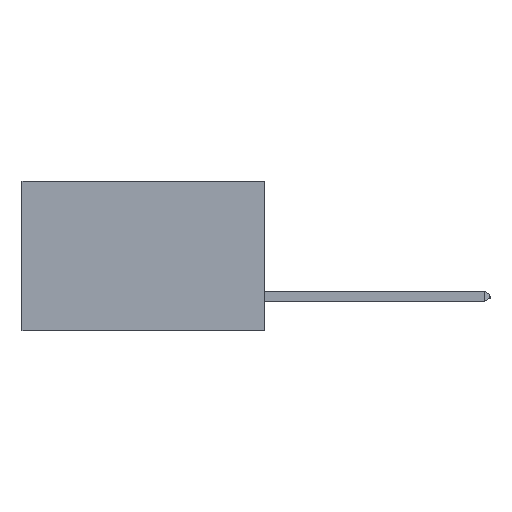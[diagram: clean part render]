
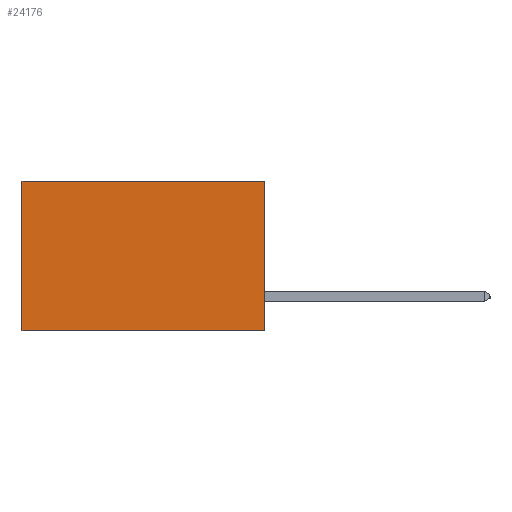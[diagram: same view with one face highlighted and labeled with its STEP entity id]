
A CAD part, left-side view. The second image highlights one B-rep face of the part: STEP entity #24176.
In plain terms, the highlighted planar face has unit normal (-1, 0, 0).
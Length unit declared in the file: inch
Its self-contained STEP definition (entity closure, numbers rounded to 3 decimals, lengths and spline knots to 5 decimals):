
#1986 = DIRECTION ( 'NONE',  ( 0., 0., -1. ) ) ;
#2754 = FACE_OUTER_BOUND ( 'NONE', #14046, .T. ) ;
#4395 = EDGE_CURVE ( 'NONE', #18801, #5040, #16166, .T. ) ;
#4834 = VERTEX_POINT ( 'NONE', #11381 ) ;
#5012 = AXIS2_PLACEMENT_3D ( 'NONE', #21224, #13677, #1986 ) ;
#5040 = VERTEX_POINT ( 'NONE', #22169 ) ;
#5149 = CARTESIAN_POINT ( 'NONE',  ( 0.298, 0., 0. ) ) ;
#5818 = EDGE_CURVE ( 'NONE', #9038, #5040, #19921, .T. ) ;
#6626 = CARTESIAN_POINT ( 'NONE',  ( 0.298, 0., -0.37 ) ) ;
#7163 = DIRECTION ( 'NONE',  ( 0., 1., 0. ) ) ;
#7274 = CARTESIAN_POINT ( 'NONE',  ( 0.298, 0., -0.37 ) ) ;
#8128 = CARTESIAN_POINT ( 'NONE',  ( 0.298, 0., 0. ) ) ;
#8557 = CARTESIAN_POINT ( 'NONE',  ( 0.298, 0.6, 0. ) ) ;
#8794 = LINE ( 'NONE', #5149, #17797 ) ;
#9038 = VERTEX_POINT ( 'NONE', #8557 ) ;
#9429 = ORIENTED_EDGE ( 'NONE', *, *, #13756, .F. ) ;
#9739 = VECTOR ( 'NONE', #14850, 39.37008 ) ;
#9760 = ORIENTED_EDGE ( 'NONE', *, *, #20472, .T. ) ;
#10057 = DIRECTION ( 'NONE',  ( 0., 0., -1. ) ) ;
#10994 = VECTOR ( 'NONE', #12097, 39.37008 ) ;
#11154 = ORIENTED_EDGE ( 'NONE', *, *, #5818, .T. ) ;
#11381 = CARTESIAN_POINT ( 'NONE',  ( 0.298, 0., 0. ) ) ;
#12097 = DIRECTION ( 'NONE',  ( 0., 1., 0. ) ) ;
#13516 = PLANE ( 'NONE',  #5012 ) ;
#13677 = DIRECTION ( 'NONE',  ( 1., 0., 0. ) ) ;
#13756 = EDGE_CURVE ( 'NONE', #4834, #18801, #24746, .T. ) ;
#14046 = EDGE_LOOP ( 'NONE', ( #11154, #21538, #9429, #9760 ) ) ;
#14843 = VECTOR ( 'NONE', #10057, 39.37008 ) ;
#14850 = DIRECTION ( 'NONE',  ( 0., 0., -1. ) ) ;
#16166 = LINE ( 'NONE', #6626, #10994 ) ;
#17797 = VECTOR ( 'NONE', #7163, 39.37008 ) ;
#18801 = VERTEX_POINT ( 'NONE', #7274 ) ;
#19921 = LINE ( 'NONE', #22224, #9739 ) ;
#20472 = EDGE_CURVE ( 'NONE', #4834, #9038, #8794, .T. ) ;
#21224 = CARTESIAN_POINT ( 'NONE',  ( 0.298, 0., 0. ) ) ;
#21538 = ORIENTED_EDGE ( 'NONE', *, *, #4395, .F. ) ;
#22169 = CARTESIAN_POINT ( 'NONE',  ( 0.298, 0.6, -0.37 ) ) ;
#22224 = CARTESIAN_POINT ( 'NONE',  ( 0.298, 0.6, 0. ) ) ;
#24176 = ADVANCED_FACE ( 'NONE', ( #2754 ), #13516, .F. ) ;
#24746 = LINE ( 'NONE', #8128, #14843 ) ;
